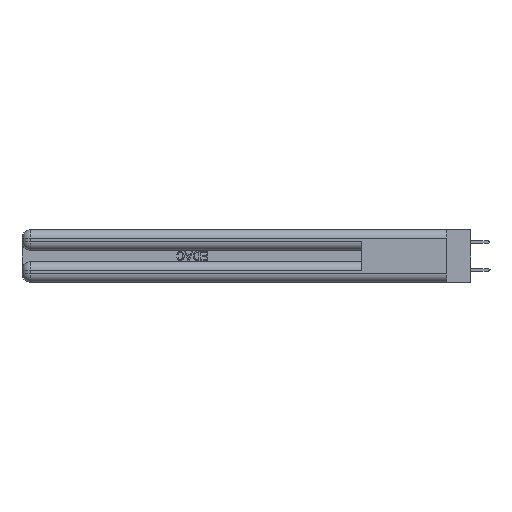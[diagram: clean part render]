
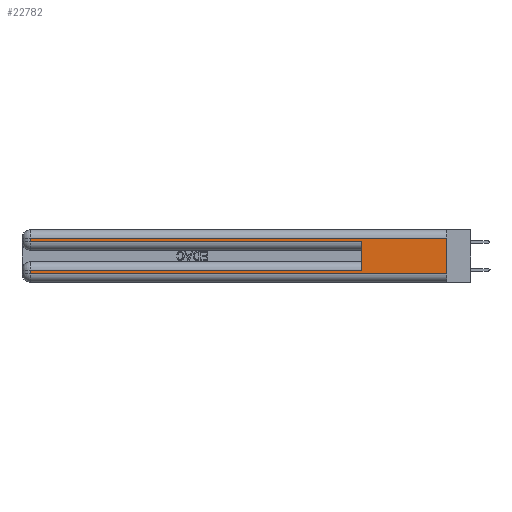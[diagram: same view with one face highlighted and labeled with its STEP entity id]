
A CAD part, left-side view. The second image highlights one B-rep face of the part: STEP entity #22782.
In plain terms, the highlighted planar face has unit normal (-1, 0, 0).
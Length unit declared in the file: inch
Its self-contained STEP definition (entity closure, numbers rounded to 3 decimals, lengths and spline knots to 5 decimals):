
#635 = ORIENTED_EDGE ( 'NONE', *, *, #38076, .T. ) ;
#786 = DIRECTION ( 'NONE',  ( 0., 0., -1. ) ) ;
#1437 = DIRECTION ( 'NONE',  ( 0., 0., -1. ) ) ;
#2077 = DIRECTION ( 'NONE',  ( 1., 0., 0. ) ) ;
#2598 = AXIS2_PLACEMENT_3D ( 'NONE', #18998, #2077, #41847 ) ;
#3824 = CARTESIAN_POINT ( 'NONE',  ( 0., 2.94, 0.085 ) ) ;
#5624 = DIRECTION ( 'NONE',  ( 0., -1., 0. ) ) ;
#5771 = EDGE_CURVE ( 'NONE', #27615, #25885, #37135, .T. ) ;
#6669 = ORIENTED_EDGE ( 'NONE', *, *, #11972, .F. ) ;
#7115 = DIRECTION ( 'NONE',  ( 0., -1., 0. ) ) ;
#7130 = EDGE_LOOP ( 'NONE', ( #28844, #31096, #29929, #38997, #6669, #635, #32876, #34429 ) ) ;
#7733 = CARTESIAN_POINT ( 'NONE',  ( 0., 2.94, 0.285 ) ) ;
#8204 = DIRECTION ( 'NONE',  ( 0., 0., 1. ) ) ;
#9095 = CARTESIAN_POINT ( 'NONE',  ( 0., 0., 0.285 ) ) ;
#9225 = PLANE ( 'NONE',  #2598 ) ;
#9954 = EDGE_CURVE ( 'NONE', #13276, #27615, #27410, .T. ) ;
#10348 = VERTEX_POINT ( 'NONE', #16690 ) ;
#10559 = CARTESIAN_POINT ( 'NONE',  ( 0., 2.94, 0.37 ) ) ;
#11642 = DIRECTION ( 'NONE',  ( 0., 1., 0. ) ) ;
#11841 = VERTEX_POINT ( 'NONE', #24940 ) ;
#11972 = EDGE_CURVE ( 'NONE', #11841, #25569, #18629, .T. ) ;
#13276 = VERTEX_POINT ( 'NONE', #3824 ) ;
#15321 = LINE ( 'NONE', #19195, #41664 ) ;
#16203 = CARTESIAN_POINT ( 'NONE',  ( 0., 2.94, 0.31 ) ) ;
#16371 = DIRECTION ( 'NONE',  ( 0., 1., 0. ) ) ;
#16690 = CARTESIAN_POINT ( 'NONE',  ( 0., 0., 0.31 ) ) ;
#17332 = LINE ( 'NONE', #18145, #35186 ) ;
#18145 = CARTESIAN_POINT ( 'NONE',  ( 0., 0., 0.31 ) ) ;
#18629 = LINE ( 'NONE', #34919, #38020 ) ;
#18998 = CARTESIAN_POINT ( 'NONE',  ( 0., 0., 0.37 ) ) ;
#19195 = CARTESIAN_POINT ( 'NONE',  ( 0., 0., 0.085 ) ) ;
#19610 = EDGE_CURVE ( 'NONE', #31288, #38655, #37092, .T. ) ;
#19683 = EDGE_CURVE ( 'NONE', #10348, #25885, #34257, .T. ) ;
#19747 = VECTOR ( 'NONE', #5624, 39.37008 ) ;
#20764 = VECTOR ( 'NONE', #7115, 39.37008 ) ;
#22694 = EDGE_CURVE ( 'NONE', #10348, #31288, #17332, .T. ) ;
#22782 = ADVANCED_FACE ( 'NONE', ( #35522 ), #9225, .F. ) ;
#23497 = DIRECTION ( 'NONE',  ( 0., 0., -1. ) ) ;
#24940 = CARTESIAN_POINT ( 'NONE',  ( 0., 0.6, 0.085 ) ) ;
#25569 = VERTEX_POINT ( 'NONE', #30767 ) ;
#25885 = VERTEX_POINT ( 'NONE', #42496 ) ;
#27140 = CARTESIAN_POINT ( 'NONE',  ( 0., 0., 0.06 ) ) ;
#27410 = LINE ( 'NONE', #39810, #34883 ) ;
#27615 = VERTEX_POINT ( 'NONE', #30096 ) ;
#28844 = ORIENTED_EDGE ( 'NONE', *, *, #19683, .F. ) ;
#29929 = ORIENTED_EDGE ( 'NONE', *, *, #19610, .T. ) ;
#30096 = CARTESIAN_POINT ( 'NONE',  ( 0., 2.94, 0.06 ) ) ;
#30767 = CARTESIAN_POINT ( 'NONE',  ( 0., 0.6, 0.285 ) ) ;
#31096 = ORIENTED_EDGE ( 'NONE', *, *, #22694, .T. ) ;
#31288 = VERTEX_POINT ( 'NONE', #16203 ) ;
#32003 = EDGE_CURVE ( 'NONE', #38655, #25569, #38893, .T. ) ;
#32876 = ORIENTED_EDGE ( 'NONE', *, *, #9954, .T. ) ;
#34257 = LINE ( 'NONE', #41869, #39868 ) ;
#34429 = ORIENTED_EDGE ( 'NONE', *, *, #5771, .T. ) ;
#34883 = VECTOR ( 'NONE', #23497, 39.37008 ) ;
#34919 = CARTESIAN_POINT ( 'NONE',  ( 0., 0.6, 0.145 ) ) ;
#35186 = VECTOR ( 'NONE', #11642, 39.37008 ) ;
#35522 = FACE_OUTER_BOUND ( 'NONE', #7130, .T. ) ;
#37092 = LINE ( 'NONE', #10559, #41248 ) ;
#37135 = LINE ( 'NONE', #27140, #20764 ) ;
#38020 = VECTOR ( 'NONE', #8204, 39.37008 ) ;
#38076 = EDGE_CURVE ( 'NONE', #11841, #13276, #15321, .T. ) ;
#38655 = VERTEX_POINT ( 'NONE', #7733 ) ;
#38893 = LINE ( 'NONE', #9095, #19747 ) ;
#38997 = ORIENTED_EDGE ( 'NONE', *, *, #32003, .T. ) ;
#39810 = CARTESIAN_POINT ( 'NONE',  ( 0., 2.94, 0.37 ) ) ;
#39868 = VECTOR ( 'NONE', #1437, 39.37008 ) ;
#41248 = VECTOR ( 'NONE', #786, 39.37008 ) ;
#41664 = VECTOR ( 'NONE', #16371, 39.37008 ) ;
#41847 = DIRECTION ( 'NONE',  ( 0., 0., -1. ) ) ;
#41869 = CARTESIAN_POINT ( 'NONE',  ( 0., 0., 0.37 ) ) ;
#42496 = CARTESIAN_POINT ( 'NONE',  ( 0., 0., 0.06 ) ) ;
